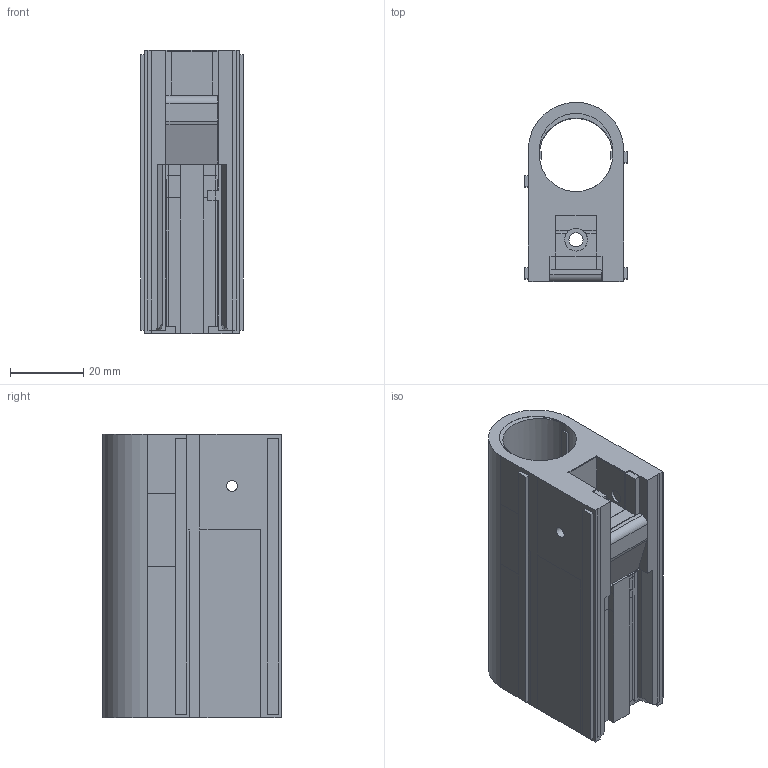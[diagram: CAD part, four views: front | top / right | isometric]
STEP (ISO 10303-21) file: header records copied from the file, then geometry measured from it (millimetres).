
FILE_DESCRIPTION(('FreeCAD Model'),'2;1');
FILE_NAME( 'ap9 bolt housing.step', '2017-11-13T22:49:07',('Author'),(''), 'Open CASCADE STEP processor 6.8','FreeCAD','Unknown');
FILE_SCHEMA(('AUTOMOTIVE_DESIGN_CC2 { 1 2 10303 214 -1 1 5 4 }'));
Length unit declared in the file: millimetre
Products named in the file (1): Pad007
Bounding box: 28 x 48.74 x 77.19 mm (x, y, z)
Volume: 44408.1 mm3; surface area: 21629.4 mm2
Topology: 1 solids, 3 shells, 239 faces, 650 edges, 421 vertices
Faces by surface type: plane 219, cylinder 20
Full cylindrical faces by diameter (mm): 2.968 x2, 3 x1, 3.566 x1, 3.861 x1, 6.25 x1, 20 x1
Entity records: 17796 total; most frequent: CARTESIAN_POINT 5049, DIRECTION 2277, LINE 1549, VECTOR 1549, ORIENTED_EDGE 1300, PCURVE 1300, DEFINITIONAL_REPRESENTATION 1300, EDGE_CURVE 650
